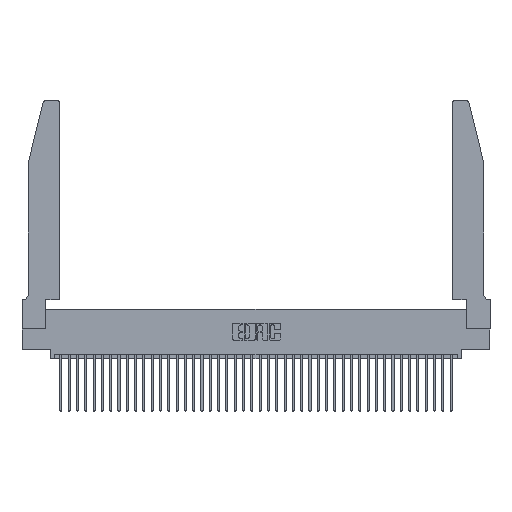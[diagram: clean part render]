
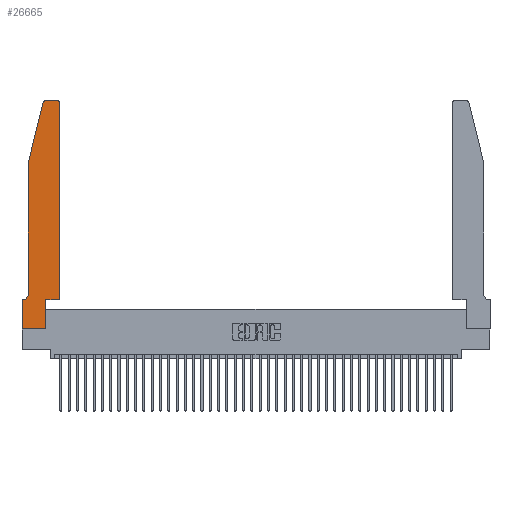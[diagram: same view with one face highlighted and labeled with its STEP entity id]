
A CAD part, top view. The second image highlights one B-rep face of the part: STEP entity #26665.
In plain terms, the highlighted planar face has unit normal (0, 0, 1).
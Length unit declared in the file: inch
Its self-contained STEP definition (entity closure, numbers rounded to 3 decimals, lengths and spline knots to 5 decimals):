
#5 = CARTESIAN_POINT ( 'NONE',  ( 0.2865, 0., 0.37 ) ) ;
#655 = CARTESIAN_POINT ( 'NONE',  ( 0.0755, 2., 0.37 ) ) ;
#1080 = CARTESIAN_POINT ( 'NONE',  ( 0.4505, 0.35, 0.37 ) ) ;
#1767 = ORIENTED_EDGE ( 'NONE', *, *, #9581, .T. ) ;
#1867 = VECTOR ( 'NONE', #41393, 39.37008 ) ;
#2543 = CARTESIAN_POINT ( 'NONE',  ( 0., 0.35, 0.37 ) ) ;
#2710 = CARTESIAN_POINT ( 'NONE',  ( 0., 0., 0.37 ) ) ;
#2742 = CARTESIAN_POINT ( 'NONE',  ( 0.284, 2.75, 0.37 ) ) ;
#2843 = DIRECTION ( 'NONE',  ( 1., 0., 0. ) ) ;
#3346 = CARTESIAN_POINT ( 'NONE',  ( 0.0755, 0.35, 0.37 ) ) ;
#3388 = ORIENTED_EDGE ( 'NONE', *, *, #7319, .T. ) ;
#3605 = CARTESIAN_POINT ( 'NONE',  ( 0.284, 2.72, 0.37 ) ) ;
#3709 = EDGE_CURVE ( 'NONE', #29800, #11358, #19428, .T. ) ;
#3910 = DIRECTION ( 'NONE',  ( 0., 1., 0. ) ) ;
#3961 = CARTESIAN_POINT ( 'NONE',  ( 0.2865, 0.35, 0.37 ) ) ;
#3980 = LINE ( 'NONE', #6194, #9630 ) ;
#4233 = EDGE_CURVE ( 'NONE', #36713, #29800, #23938, .T. ) ;
#4613 = EDGE_CURVE ( 'NONE', #23984, #27886, #10682, .T. ) ;
#4622 = VECTOR ( 'NONE', #11073, 39.37008 ) ;
#4645 = EDGE_CURVE ( 'NONE', #28015, #39179, #3980, .T. ) ;
#5464 = CARTESIAN_POINT ( 'NONE',  ( 0., 0., 0.37 ) ) ;
#5579 = VERTEX_POINT ( 'NONE', #39289 ) ;
#6194 = CARTESIAN_POINT ( 'NONE',  ( 0.4505, 0.35, 0.37 ) ) ;
#6557 = DIRECTION ( 'NONE',  ( 0., -1., 0. ) ) ;
#6655 = ORIENTED_EDGE ( 'NONE', *, *, #4233, .T. ) ;
#6953 = DIRECTION ( 'NONE',  ( 1., 0., 0. ) ) ;
#7319 = EDGE_CURVE ( 'NONE', #26555, #30425, #27706, .T. ) ;
#7457 = CARTESIAN_POINT ( 'NONE',  ( 0.0055, 0.42, 0.37 ) ) ;
#7646 = CIRCLE ( 'NONE', #13176, 0.03 ) ;
#7912 = VECTOR ( 'NONE', #3910, 39.37008 ) ;
#7933 = ORIENTED_EDGE ( 'NONE', *, *, #4613, .T. ) ;
#8315 = EDGE_CURVE ( 'NONE', #11358, #28196, #10012, .T. ) ;
#8938 = LINE ( 'NONE', #17157, #7912 ) ;
#8972 = VERTEX_POINT ( 'NONE', #35370 ) ;
#9188 = DIRECTION ( 'NONE',  ( 0., 0., 1. ) ) ;
#9311 = ORIENTED_EDGE ( 'NONE', *, *, #38539, .T. ) ;
#9581 = EDGE_CURVE ( 'NONE', #8972, #23984, #30072, .T. ) ;
#9630 = VECTOR ( 'NONE', #2843, 39.37008 ) ;
#10012 = LINE ( 'NONE', #3346, #34656 ) ;
#10051 = ORIENTED_EDGE ( 'NONE', *, *, #11438, .T. ) ;
#10151 = ORIENTED_EDGE ( 'NONE', *, *, #4645, .T. ) ;
#10682 = LINE ( 'NONE', #15964, #1867 ) ;
#10775 = DIRECTION ( 'NONE',  ( -1., 0., 0. ) ) ;
#10866 = ORIENTED_EDGE ( 'NONE', *, *, #30991, .T. ) ;
#11073 = DIRECTION ( 'NONE',  ( 0., 1., 0. ) ) ;
#11358 = VERTEX_POINT ( 'NONE', #13957 ) ;
#11438 = EDGE_CURVE ( 'NONE', #39179, #8972, #13417, .T. ) ;
#13176 = AXIS2_PLACEMENT_3D ( 'NONE', #3605, #26377, #6953 ) ;
#13417 = LINE ( 'NONE', #1080, #4622 ) ;
#13794 = LINE ( 'NONE', #655, #28832 ) ;
#13957 = CARTESIAN_POINT ( 'NONE',  ( 0.0055, 0.35, 0.37 ) ) ;
#15964 = CARTESIAN_POINT ( 'NONE',  ( 0.2605, 2.75, 0.37 ) ) ;
#16643 = CARTESIAN_POINT ( 'NONE',  ( 0., 0., 0.37 ) ) ;
#17157 = CARTESIAN_POINT ( 'NONE',  ( 0.2865, 0.35, 0.37 ) ) ;
#18397 = AXIS2_PLACEMENT_3D ( 'NONE', #2543, #9188, #31771 ) ;
#18972 = CARTESIAN_POINT ( 'NONE',  ( 0.4205, 2.75, 0.37 ) ) ;
#19166 = DIRECTION ( 'NONE',  ( 0., 0., 1. ) ) ;
#19225 = DIRECTION ( 'NONE',  ( 0., -1., 0. ) ) ;
#19428 = CIRCLE ( 'NONE', #30389, 0.07 ) ;
#22243 = FACE_OUTER_BOUND ( 'NONE', #26493, .T. ) ;
#22544 = LINE ( 'NONE', #2710, #29983 ) ;
#22948 = DIRECTION ( 'NONE',  ( -1., 0., 0. ) ) ;
#22981 = ORIENTED_EDGE ( 'NONE', *, *, #3709, .T. ) ;
#23124 = DIRECTION ( 'NONE',  ( 1., 0., 0. ) ) ;
#23938 = LINE ( 'NONE', #26011, #31368 ) ;
#23984 = VERTEX_POINT ( 'NONE', #18972 ) ;
#24175 = EDGE_CURVE ( 'NONE', #27886, #5579, #7646, .T. ) ;
#26011 = CARTESIAN_POINT ( 'NONE',  ( 0.0755, 2., 0.37 ) ) ;
#26377 = DIRECTION ( 'NONE',  ( 0., 0., 1. ) ) ;
#26493 = EDGE_LOOP ( 'NONE', ( #7933, #31109, #9311, #6655, #22981, #26848, #10866, #3388, #26659, #10151, #10051, #1767 ) ) ;
#26555 = VERTEX_POINT ( 'NONE', #5464 ) ;
#26659 = ORIENTED_EDGE ( 'NONE', *, *, #28143, .T. ) ;
#26665 = ADVANCED_FACE ( 'NONE', ( #22243 ), #31637, .T. ) ;
#26787 = CARTESIAN_POINT ( 'NONE',  ( 0., 0.35, 0.37 ) ) ;
#26848 = ORIENTED_EDGE ( 'NONE', *, *, #8315, .T. ) ;
#27706 = LINE ( 'NONE', #16643, #33189 ) ;
#27886 = VERTEX_POINT ( 'NONE', #2742 ) ;
#28015 = VERTEX_POINT ( 'NONE', #3961 ) ;
#28143 = EDGE_CURVE ( 'NONE', #30425, #28015, #8938, .T. ) ;
#28196 = VERTEX_POINT ( 'NONE', #26787 ) ;
#28832 = VECTOR ( 'NONE', #33029, 39.37008 ) ;
#29765 = CARTESIAN_POINT ( 'NONE',  ( 0.4505, 0.35, 0.37 ) ) ;
#29800 = VERTEX_POINT ( 'NONE', #32152 ) ;
#29983 = VECTOR ( 'NONE', #19225, 39.37008 ) ;
#30070 = DIRECTION ( 'NONE',  ( 0., 0., -1. ) ) ;
#30072 = CIRCLE ( 'NONE', #35316, 0.03 ) ;
#30389 = AXIS2_PLACEMENT_3D ( 'NONE', #7457, #30070, #10775 ) ;
#30425 = VERTEX_POINT ( 'NONE', #5 ) ;
#30991 = EDGE_CURVE ( 'NONE', #28196, #26555, #22544, .T. ) ;
#31109 = ORIENTED_EDGE ( 'NONE', *, *, #24175, .T. ) ;
#31368 = VECTOR ( 'NONE', #6557, 39.37008 ) ;
#31637 = PLANE ( 'NONE',  #18397 ) ;
#31771 = DIRECTION ( 'NONE',  ( 1., 0., 0. ) ) ;
#32152 = CARTESIAN_POINT ( 'NONE',  ( 0.0755, 0.42, 0.37 ) ) ;
#33029 = DIRECTION ( 'NONE',  ( -0.239, -0.971, 0. ) ) ;
#33189 = VECTOR ( 'NONE', #23124, 39.37008 ) ;
#34656 = VECTOR ( 'NONE', #22948, 39.37008 ) ;
#35316 = AXIS2_PLACEMENT_3D ( 'NONE', #38239, #19166, #41361 ) ;
#35370 = CARTESIAN_POINT ( 'NONE',  ( 0.4505, 2.72, 0.37 ) ) ;
#36713 = VERTEX_POINT ( 'NONE', #40151 ) ;
#38239 = CARTESIAN_POINT ( 'NONE',  ( 0.4205, 2.72, 0.37 ) ) ;
#38539 = EDGE_CURVE ( 'NONE', #5579, #36713, #13794, .T. ) ;
#39179 = VERTEX_POINT ( 'NONE', #29765 ) ;
#39289 = CARTESIAN_POINT ( 'NONE',  ( 0.25487, 2.72718, 0.37 ) ) ;
#40151 = CARTESIAN_POINT ( 'NONE',  ( 0.0755, 2., 0.37 ) ) ;
#41361 = DIRECTION ( 'NONE',  ( 1., 0., 0. ) ) ;
#41393 = DIRECTION ( 'NONE',  ( -1., 0., 0. ) ) ;
